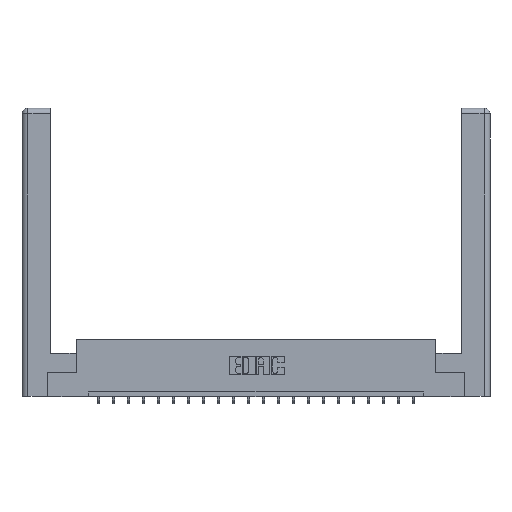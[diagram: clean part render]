
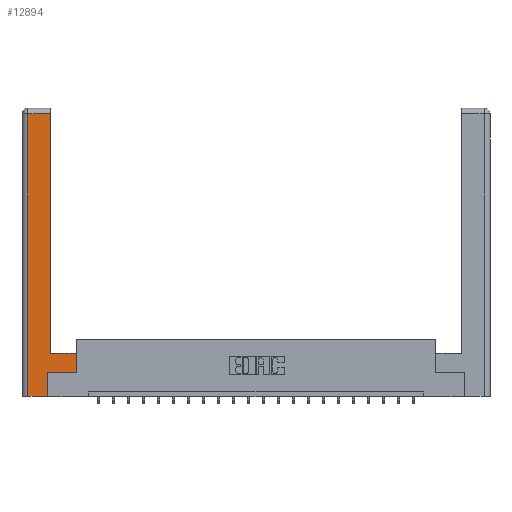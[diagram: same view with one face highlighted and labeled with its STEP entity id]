
A CAD part, top view. The second image highlights one B-rep face of the part: STEP entity #12894.
In plain terms, the highlighted planar face has unit normal (0, 0, 1).
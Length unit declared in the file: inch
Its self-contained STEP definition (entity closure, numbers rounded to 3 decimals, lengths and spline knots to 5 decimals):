
#101 = DIRECTION ( 'NONE',  ( 1., 0., 0. ) ) ;
#350 = CARTESIAN_POINT ( 'NONE',  ( 0.265, 0.245, 0. ) ) ;
#840 = DIRECTION ( 'NONE',  ( -1., 0., 0. ) ) ;
#1167 = CARTESIAN_POINT ( 'NONE',  ( 0.265, 0., 0. ) ) ;
#1396 = ORIENTED_EDGE ( 'NONE', *, *, #1661, .T. ) ;
#1490 = DIRECTION ( 'NONE',  ( -1., 0., 0. ) ) ;
#1661 = EDGE_CURVE ( 'NONE', #17672, #7682, #4008, .T. ) ;
#2611 = DIRECTION ( 'NONE',  ( 0., -1., 0. ) ) ;
#2722 = EDGE_CURVE ( 'NONE', #6848, #4923, #7868, .T. ) ;
#2820 = VECTOR ( 'NONE', #4577, 39.37008 ) ;
#3110 = ORIENTED_EDGE ( 'NONE', *, *, #11741, .T. ) ;
#3470 = CARTESIAN_POINT ( 'NONE',  ( 0.0615, 2.94, 0. ) ) ;
#4008 = LINE ( 'NONE', #19887, #9736 ) ;
#4577 = DIRECTION ( 'NONE',  ( 0., 1., 0. ) ) ;
#4923 = VERTEX_POINT ( 'NONE', #13553 ) ;
#5466 = CARTESIAN_POINT ( 'NONE',  ( 0.265, 0., 0. ) ) ;
#5785 = DIRECTION ( 'NONE',  ( 0., 1., 0. ) ) ;
#6848 = VERTEX_POINT ( 'NONE', #3470 ) ;
#7065 = VERTEX_POINT ( 'NONE', #19249 ) ;
#7252 = LINE ( 'NONE', #19565, #2820 ) ;
#7677 = VECTOR ( 'NONE', #1490, 39.37008 ) ;
#7682 = VERTEX_POINT ( 'NONE', #12012 ) ;
#7868 = LINE ( 'NONE', #12591, #12809 ) ;
#8262 = LINE ( 'NONE', #11574, #12682 ) ;
#8274 = CARTESIAN_POINT ( 'NONE',  ( 0.0615, 2.94, 0. ) ) ;
#8423 = EDGE_CURVE ( 'NONE', #15428, #17556, #19713, .T. ) ;
#8530 = LINE ( 'NONE', #1167, #12410 ) ;
#9720 = VECTOR ( 'NONE', #5785, 39.37008 ) ;
#9736 = VECTOR ( 'NONE', #14640, 39.37008 ) ;
#9812 = VERTEX_POINT ( 'NONE', #19920 ) ;
#10359 = DIRECTION ( 'NONE',  ( -1., 0., 0. ) ) ;
#11574 = CARTESIAN_POINT ( 'NONE',  ( 0.565, 0.245, 0. ) ) ;
#11741 = EDGE_CURVE ( 'NONE', #4923, #15428, #8530, .T. ) ;
#12012 = CARTESIAN_POINT ( 'NONE',  ( 0.565, 0.45, 0. ) ) ;
#12279 = PLANE ( 'NONE',  #19187 ) ;
#12410 = VECTOR ( 'NONE', #101, 39.37008 ) ;
#12591 = CARTESIAN_POINT ( 'NONE',  ( 0.0615, 0., 0. ) ) ;
#12682 = VECTOR ( 'NONE', #21566, 39.37008 ) ;
#12809 = VECTOR ( 'NONE', #2611, 39.37008 ) ;
#12894 = ADVANCED_FACE ( 'NONE', ( #16717 ), #12279, .F. ) ;
#13446 = EDGE_CURVE ( 'NONE', #9812, #7065, #7252, .T. ) ;
#13553 = CARTESIAN_POINT ( 'NONE',  ( 0.0615, 0., 0. ) ) ;
#13985 = EDGE_CURVE ( 'NONE', #17556, #17672, #8262, .T. ) ;
#14131 = ORIENTED_EDGE ( 'NONE', *, *, #19550, .T. ) ;
#14248 = CARTESIAN_POINT ( 'NONE',  ( 0.565, 0.245, 0. ) ) ;
#14640 = DIRECTION ( 'NONE',  ( 0., 1., 0. ) ) ;
#15428 = VERTEX_POINT ( 'NONE', #5466 ) ;
#15658 = CARTESIAN_POINT ( 'NONE',  ( 0., 0., 0. ) ) ;
#15818 = EDGE_CURVE ( 'NONE', #7065, #6848, #21041, .T. ) ;
#16717 = FACE_OUTER_BOUND ( 'NONE', #18428, .T. ) ;
#17381 = DIRECTION ( 'NONE',  ( 0., 0., -1. ) ) ;
#17556 = VERTEX_POINT ( 'NONE', #350 ) ;
#17672 = VERTEX_POINT ( 'NONE', #14248 ) ;
#18039 = LINE ( 'NONE', #20644, #19348 ) ;
#18428 = EDGE_LOOP ( 'NONE', ( #18842, #20774, #19888, #3110, #19429, #21516, #1396, #14131 ) ) ;
#18842 = ORIENTED_EDGE ( 'NONE', *, *, #13446, .T. ) ;
#19040 = CARTESIAN_POINT ( 'NONE',  ( 0.265, 0.245, 0. ) ) ;
#19187 = AXIS2_PLACEMENT_3D ( 'NONE', #15658, #17381, #840 ) ;
#19249 = CARTESIAN_POINT ( 'NONE',  ( 0.295, 2.94, 0. ) ) ;
#19348 = VECTOR ( 'NONE', #10359, 39.37008 ) ;
#19429 = ORIENTED_EDGE ( 'NONE', *, *, #8423, .T. ) ;
#19550 = EDGE_CURVE ( 'NONE', #7682, #9812, #18039, .T. ) ;
#19565 = CARTESIAN_POINT ( 'NONE',  ( 0.295, 3., 0. ) ) ;
#19713 = LINE ( 'NONE', #19040, #9720 ) ;
#19887 = CARTESIAN_POINT ( 'NONE',  ( 0.565, 0.45, 0. ) ) ;
#19888 = ORIENTED_EDGE ( 'NONE', *, *, #2722, .T. ) ;
#19920 = CARTESIAN_POINT ( 'NONE',  ( 0.295, 0.45, 0. ) ) ;
#20644 = CARTESIAN_POINT ( 'NONE',  ( 0.295, 0.45, 0. ) ) ;
#20774 = ORIENTED_EDGE ( 'NONE', *, *, #15818, .T. ) ;
#21041 = LINE ( 'NONE', #8274, #7677 ) ;
#21516 = ORIENTED_EDGE ( 'NONE', *, *, #13985, .T. ) ;
#21566 = DIRECTION ( 'NONE',  ( 1., 0., 0. ) ) ;
